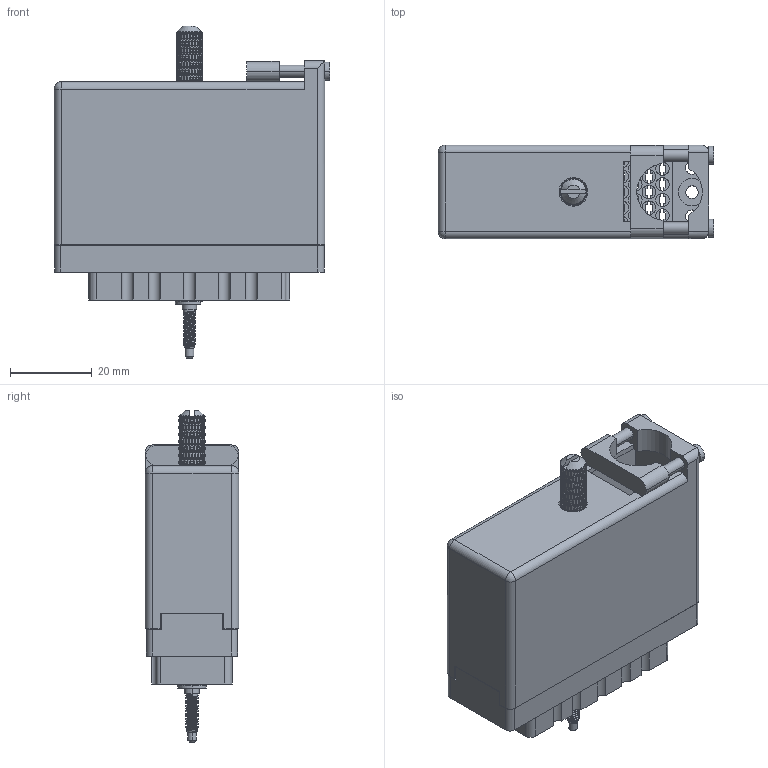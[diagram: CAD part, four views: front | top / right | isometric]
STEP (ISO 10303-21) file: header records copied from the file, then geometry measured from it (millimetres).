
FILE_DESCRIPTION (( 'STEP AP203' ), '1' );
FILE_NAME ('516-056-000-265.STEP', '2020-03-05T19:49:55', ( '' ), ( '' ), 'SwSTEP 2.0', 'SolidWorks 2016', '' );
FILE_SCHEMA (( 'CONFIG_CONTROL_DESIGN' ));
Length unit declared in the file: inch
Products named in the file (8): 516-230-001_Metal - 056 Top Entry; 516-253-138-107; 516-056-000-265; 516 Part Receptacle_056; 516-250-038-111; 516-253-035-100; 516-251-035-100; Actuating Screw Assy 038-056
Assembly tree (8 placements, depth 3):
  516-056-000-265
    516 Part Receptacle_056
    516-230-001_Metal - 056 Top Entry
    Actuating Screw Assy 038-056
      516-251-035-100
      516-253-035-100  x2
      516-253-138-107
      516-250-038-111
Bounding box: 67.31 x 22.83 x 81.03 mm (x, y, z)
Volume: 26674.5 mm3; surface area: 38469.5 mm2
Topology: 7 solids, 7 shells, 2729 faces, 6916 edges, 4218 vertices
Faces by surface type: bspline 1006, plane 1002, cylinder 699, cone 20, sphere 2
Entity records: 111693 total; most frequent: CARTESIAN_POINT 56052, ORIENTED_EDGE 13804, DIRECTION 8901, EDGE_CURVE 6902, VERTEX_POINT 4210, LINE 3003, VECTOR 3003, AXIS2_PLACEMENT_3D 2949
